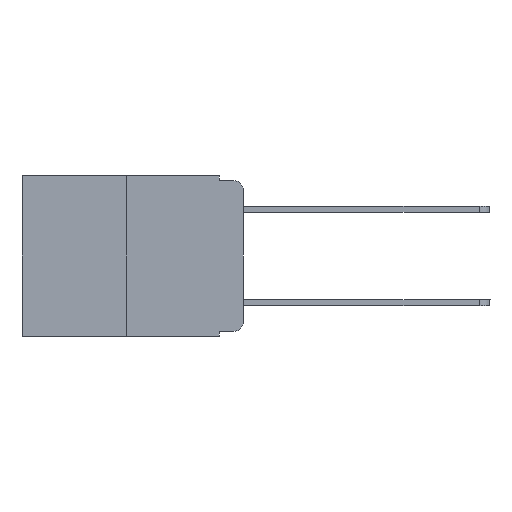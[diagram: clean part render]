
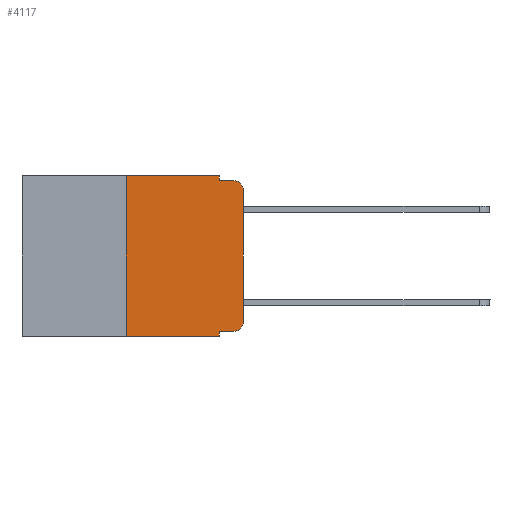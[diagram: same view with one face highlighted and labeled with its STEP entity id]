
A CAD part, left-side view. The second image highlights one B-rep face of the part: STEP entity #4117.
In plain terms, the highlighted planar face has unit normal (-1, 0, 0).
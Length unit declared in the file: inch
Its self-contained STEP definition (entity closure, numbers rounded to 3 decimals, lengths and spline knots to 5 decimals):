
#217 = VECTOR ( 'NONE', #6970, 39.37008 ) ;
#459 = CARTESIAN_POINT ( 'NONE',  ( 0., 0.051, -0.333 ) ) ;
#602 = CARTESIAN_POINT ( 'NONE',  ( 0., 0., -0.313 ) ) ;
#625 = DIRECTION ( 'NONE',  ( 0., 0., 1. ) ) ;
#627 = VECTOR ( 'NONE', #4396, 39.37008 ) ;
#671 = DIRECTION ( 'NONE',  ( 1., 0., 0. ) ) ;
#686 = EDGE_CURVE ( 'NONE', #4932, #3060, #10999, .T. ) ;
#744 = CIRCLE ( 'NONE', #7586, 0.02 ) ;
#895 = ORIENTED_EDGE ( 'NONE', *, *, #686, .F. ) ;
#1423 = EDGE_CURVE ( 'NONE', #6611, #7618, #7644, .T. ) ;
#1500 = DIRECTION ( 'NONE',  ( 0., 0., -1. ) ) ;
#1577 = EDGE_CURVE ( 'NONE', #7618, #8928, #6636, .T. ) ;
#1789 = DIRECTION ( 'NONE',  ( 0., 0., -1. ) ) ;
#1996 = AXIS2_PLACEMENT_3D ( 'NONE', #8950, #671, #8007 ) ;
#2490 = EDGE_CURVE ( 'NONE', #8928, #10521, #9053, .T. ) ;
#2511 = DIRECTION ( 'NONE',  ( 0., 0., 1. ) ) ;
#2780 = ORIENTED_EDGE ( 'NONE', *, *, #2490, .T. ) ;
#2783 = CARTESIAN_POINT ( 'NONE',  ( 0., 0.051, 0. ) ) ;
#2911 = ORIENTED_EDGE ( 'NONE', *, *, #9049, .F. ) ;
#2950 = EDGE_CURVE ( 'NONE', #7423, #3397, #10371, .T. ) ;
#3045 = DIRECTION ( 'NONE',  ( 0., -1., 0. ) ) ;
#3060 = VERTEX_POINT ( 'NONE', #5063 ) ;
#3235 = ORIENTED_EDGE ( 'NONE', *, *, #5709, .F. ) ;
#3382 = ORIENTED_EDGE ( 'NONE', *, *, #1577, .T. ) ;
#3397 = VERTEX_POINT ( 'NONE', #9653 ) ;
#3578 = VECTOR ( 'NONE', #3045, 39.37008 ) ;
#3830 = VECTOR ( 'NONE', #625, 39.37008 ) ;
#4117 = ADVANCED_FACE ( 'NONE', ( #4206 ), #6235, .F. ) ;
#4206 = FACE_OUTER_BOUND ( 'NONE', #6066, .T. ) ;
#4212 = CARTESIAN_POINT ( 'NONE',  ( 0., 0.02, -0.03 ) ) ;
#4396 = DIRECTION ( 'NONE',  ( 0., 0., -1. ) ) ;
#4932 = VERTEX_POINT ( 'NONE', #7456 ) ;
#5063 = CARTESIAN_POINT ( 'NONE',  ( 0., 0.02, -0.01 ) ) ;
#5128 = VECTOR ( 'NONE', #1789, 39.37008 ) ;
#5167 = DIRECTION ( 'NONE',  ( 0., 0., -1. ) ) ;
#5285 = CARTESIAN_POINT ( 'NONE',  ( 0., 0.25, 0. ) ) ;
#5428 = VERTEX_POINT ( 'NONE', #6043 ) ;
#5486 = ORIENTED_EDGE ( 'NONE', *, *, #9493, .T. ) ;
#5533 = CARTESIAN_POINT ( 'NONE',  ( 0., 0.473, 0. ) ) ;
#5709 = EDGE_CURVE ( 'NONE', #7423, #10045, #10297, .T. ) ;
#5922 = ORIENTED_EDGE ( 'NONE', *, *, #1423, .T. ) ;
#5958 = VECTOR ( 'NONE', #6464, 39.37008 ) ;
#6043 = CARTESIAN_POINT ( 'NONE',  ( 0., 0.051, 0. ) ) ;
#6066 = EDGE_LOOP ( 'NONE', ( #2780, #5486, #895, #8927, #8764, #3235, #8443, #2911, #5922, #3382 ) ) ;
#6090 = VECTOR ( 'NONE', #2511, 39.37008 ) ;
#6235 = PLANE ( 'NONE',  #1996 ) ;
#6464 = DIRECTION ( 'NONE',  ( 0., -1., 0. ) ) ;
#6611 = VERTEX_POINT ( 'NONE', #12019 ) ;
#6636 = CIRCLE ( 'NONE', #10988, 0.02 ) ;
#6720 = CARTESIAN_POINT ( 'NONE',  ( 0., 0., -0.03 ) ) ;
#6748 = CARTESIAN_POINT ( 'NONE',  ( 0., 0.051, -0.01 ) ) ;
#6970 = DIRECTION ( 'NONE',  ( 0., -1., 0. ) ) ;
#7048 = DIRECTION ( 'NONE',  ( -1., 0., 0. ) ) ;
#7423 = VERTEX_POINT ( 'NONE', #7591 ) ;
#7456 = CARTESIAN_POINT ( 'NONE',  ( 0., 0.051, -0.01 ) ) ;
#7586 = AXIS2_PLACEMENT_3D ( 'NONE', #4212, #9758, #1500 ) ;
#7591 = CARTESIAN_POINT ( 'NONE',  ( 0., 0.25, -0.343 ) ) ;
#7618 = VERTEX_POINT ( 'NONE', #9527 ) ;
#7644 = LINE ( 'NONE', #459, #217 ) ;
#8007 = DIRECTION ( 'NONE',  ( 0., 0., -1. ) ) ;
#8020 = LINE ( 'NONE', #11788, #627 ) ;
#8072 = CARTESIAN_POINT ( 'NONE',  ( 0., 0.25, 0. ) ) ;
#8124 = CARTESIAN_POINT ( 'NONE',  ( 0., 0.02, -0.313 ) ) ;
#8443 = ORIENTED_EDGE ( 'NONE', *, *, #2950, .T. ) ;
#8764 = ORIENTED_EDGE ( 'NONE', *, *, #10305, .F. ) ;
#8768 = LINE ( 'NONE', #2783, #5128 ) ;
#8814 = DIRECTION ( 'NONE',  ( 0., -1., 0. ) ) ;
#8927 = ORIENTED_EDGE ( 'NONE', *, *, #8929, .F. ) ;
#8928 = VERTEX_POINT ( 'NONE', #602 ) ;
#8929 = EDGE_CURVE ( 'NONE', #5428, #4932, #8020, .T. ) ;
#8950 = CARTESIAN_POINT ( 'NONE',  ( 0., 0.473, 0. ) ) ;
#9049 = EDGE_CURVE ( 'NONE', #6611, #3397, #8768, .T. ) ;
#9053 = LINE ( 'NONE', #11720, #3830 ) ;
#9493 = EDGE_CURVE ( 'NONE', #10521, #3060, #744, .T. ) ;
#9527 = CARTESIAN_POINT ( 'NONE',  ( 0., 0.02, -0.333 ) ) ;
#9653 = CARTESIAN_POINT ( 'NONE',  ( 0., 0.051, -0.343 ) ) ;
#9758 = DIRECTION ( 'NONE',  ( -1., 0., 0. ) ) ;
#10045 = VERTEX_POINT ( 'NONE', #5285 ) ;
#10297 = LINE ( 'NONE', #8072, #6090 ) ;
#10305 = EDGE_CURVE ( 'NONE', #10045, #5428, #10894, .T. ) ;
#10371 = LINE ( 'NONE', #10725, #10944 ) ;
#10521 = VERTEX_POINT ( 'NONE', #6720 ) ;
#10725 = CARTESIAN_POINT ( 'NONE',  ( 0., 0.473, -0.343 ) ) ;
#10894 = LINE ( 'NONE', #5533, #5958 ) ;
#10944 = VECTOR ( 'NONE', #8814, 39.37008 ) ;
#10988 = AXIS2_PLACEMENT_3D ( 'NONE', #8124, #7048, #5167 ) ;
#10999 = LINE ( 'NONE', #6748, #3578 ) ;
#11720 = CARTESIAN_POINT ( 'NONE',  ( 0., 0., 0. ) ) ;
#11788 = CARTESIAN_POINT ( 'NONE',  ( 0., 0.051, 0. ) ) ;
#12019 = CARTESIAN_POINT ( 'NONE',  ( 0., 0.051, -0.333 ) ) ;
